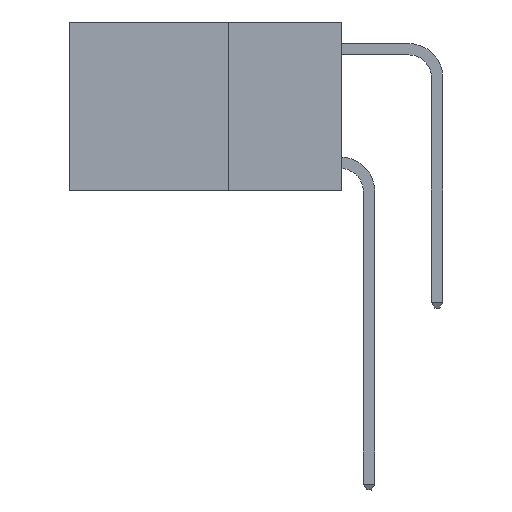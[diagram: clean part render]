
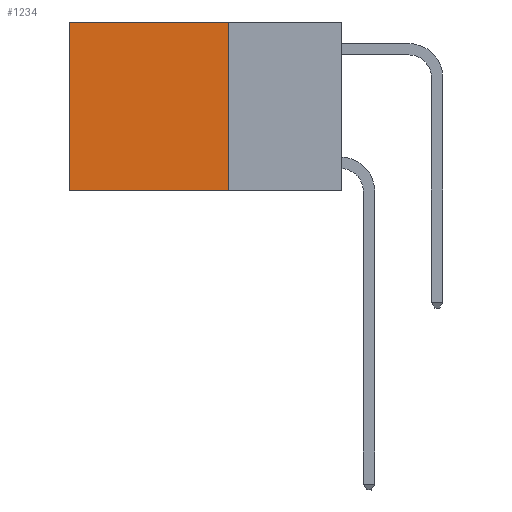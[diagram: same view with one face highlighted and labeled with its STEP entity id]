
A CAD part, left-side view. The second image highlights one B-rep face of the part: STEP entity #1234.
In plain terms, the highlighted planar face has unit normal (-1, 0, 0).
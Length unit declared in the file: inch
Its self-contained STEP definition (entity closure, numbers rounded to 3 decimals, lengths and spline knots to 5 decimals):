
#92 = DIRECTION ( 'NONE',  ( 1., 0., 0. ) ) ;
#253 = LINE ( 'NONE', #8696, #9898 ) ;
#374 = LINE ( 'NONE', #20334, #9761 ) ;
#1234 = ADVANCED_FACE ( 'NONE', ( #16467 ), #10922, .F. ) ;
#1263 = VERTEX_POINT ( 'NONE', #20814 ) ;
#1355 = ORIENTED_EDGE ( 'NONE', *, *, #11499, .T. ) ;
#1420 = LINE ( 'NONE', #11134, #10259 ) ;
#3161 = CARTESIAN_POINT ( 'NONE',  ( 0.2625, 0.6, 0. ) ) ;
#3178 = DIRECTION ( 'NONE',  ( 0., 1., 0. ) ) ;
#3502 = CARTESIAN_POINT ( 'NONE',  ( 0.2625, 0.25, 0. ) ) ;
#4126 = EDGE_CURVE ( 'NONE', #20040, #10815, #374, .T. ) ;
#4808 = ORIENTED_EDGE ( 'NONE', *, *, #4126, .F. ) ;
#5706 = DIRECTION ( 'NONE',  ( 0., 0., -1. ) ) ;
#6242 = VECTOR ( 'NONE', #3178, 39.37008 ) ;
#7057 = VERTEX_POINT ( 'NONE', #3161 ) ;
#8175 = DIRECTION ( 'NONE',  ( 0., 1., 0. ) ) ;
#8696 = CARTESIAN_POINT ( 'NONE',  ( 0.2625, 0.6, 0. ) ) ;
#8725 = CARTESIAN_POINT ( 'NONE',  ( 0.2625, 0.25, -0.37 ) ) ;
#9761 = VECTOR ( 'NONE', #17056, 39.37008 ) ;
#9898 = VECTOR ( 'NONE', #5706, 39.37008 ) ;
#9904 = ORIENTED_EDGE ( 'NONE', *, *, #17977, .T. ) ;
#10259 = VECTOR ( 'NONE', #8175, 39.37008 ) ;
#10815 = VERTEX_POINT ( 'NONE', #8725 ) ;
#10922 = PLANE ( 'NONE',  #14705 ) ;
#11053 = LINE ( 'NONE', #20796, #6242 ) ;
#11134 = CARTESIAN_POINT ( 'NONE',  ( 0.2625, 0.25, 0. ) ) ;
#11353 = DIRECTION ( 'NONE',  ( 0., 0., -1. ) ) ;
#11499 = EDGE_CURVE ( 'NONE', #7057, #1263, #253, .T. ) ;
#13737 = EDGE_CURVE ( 'NONE', #10815, #1263, #11053, .T. ) ;
#14147 = CARTESIAN_POINT ( 'NONE',  ( 0.2625, 0.25, 0. ) ) ;
#14705 = AXIS2_PLACEMENT_3D ( 'NONE', #14147, #92, #11353 ) ;
#16467 = FACE_OUTER_BOUND ( 'NONE', #17900, .T. ) ;
#17056 = DIRECTION ( 'NONE',  ( 0., 0., -1. ) ) ;
#17900 = EDGE_LOOP ( 'NONE', ( #1355, #20003, #4808, #9904 ) ) ;
#17977 = EDGE_CURVE ( 'NONE', #20040, #7057, #1420, .T. ) ;
#20003 = ORIENTED_EDGE ( 'NONE', *, *, #13737, .F. ) ;
#20040 = VERTEX_POINT ( 'NONE', #3502 ) ;
#20334 = CARTESIAN_POINT ( 'NONE',  ( 0.2625, 0.25, 0. ) ) ;
#20796 = CARTESIAN_POINT ( 'NONE',  ( 0.2625, 0.25, -0.37 ) ) ;
#20814 = CARTESIAN_POINT ( 'NONE',  ( 0.2625, 0.6, -0.37 ) ) ;
